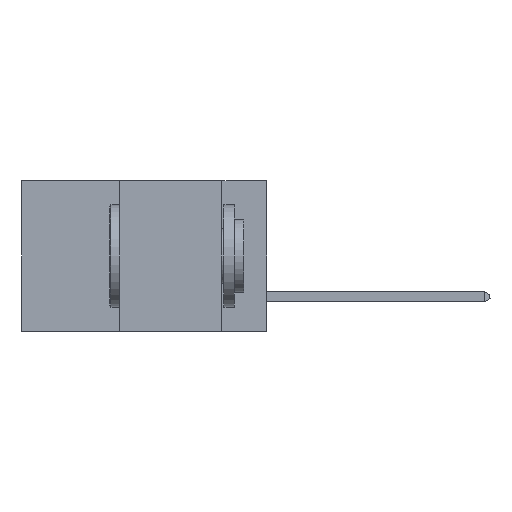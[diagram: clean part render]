
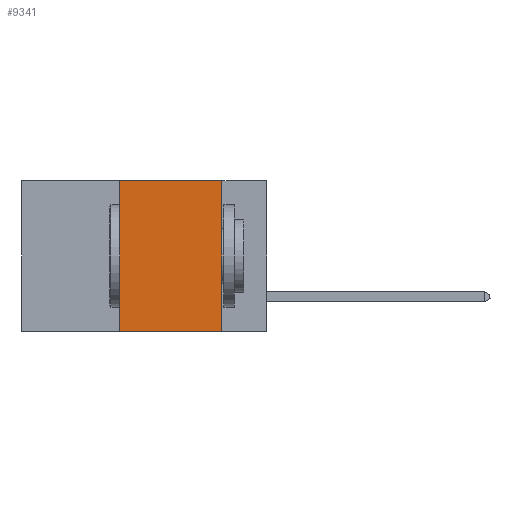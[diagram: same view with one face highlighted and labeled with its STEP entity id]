
A CAD part, left-side view. The second image highlights one B-rep face of the part: STEP entity #9341.
In plain terms, the highlighted planar face has unit normal (-1, 0, 0).
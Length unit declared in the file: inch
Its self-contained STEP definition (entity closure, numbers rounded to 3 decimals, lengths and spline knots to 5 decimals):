
#2614 = FACE_OUTER_BOUND ( 'NONE', #15509, .T. ) ;
#2659 = DIRECTION ( 'NONE',  ( 0., -1., 0. ) ) ;
#3220 = CARTESIAN_POINT ( 'NONE',  ( 0., 0.11, -0.37 ) ) ;
#4090 = DIRECTION ( 'NONE',  ( 0., 0., -1. ) ) ;
#4826 = CARTESIAN_POINT ( 'NONE',  ( 0., 0.36, -0.37 ) ) ;
#5316 = VERTEX_POINT ( 'NONE', #4826 ) ;
#5950 = VECTOR ( 'NONE', #25787, 39.37008 ) ;
#6072 = CARTESIAN_POINT ( 'NONE',  ( 0., 0.6, 0. ) ) ;
#6978 = LINE ( 'NONE', #11052, #22862 ) ;
#7278 = EDGE_CURVE ( 'NONE', #8831, #9367, #6978, .T. ) ;
#8831 = VERTEX_POINT ( 'NONE', #9322 ) ;
#9322 = CARTESIAN_POINT ( 'NONE',  ( 0., 0.36, 0. ) ) ;
#9341 = ADVANCED_FACE ( 'NONE', ( #2614 ), #10230, .F. ) ;
#9367 = VERTEX_POINT ( 'NONE', #18439 ) ;
#10228 = VECTOR ( 'NONE', #10442, 39.37008 ) ;
#10230 = PLANE ( 'NONE',  #13656 ) ;
#10442 = DIRECTION ( 'NONE',  ( 0., 0., 1. ) ) ;
#11052 = CARTESIAN_POINT ( 'NONE',  ( 0., 0.6, 0. ) ) ;
#11776 = EDGE_CURVE ( 'NONE', #5316, #24191, #11885, .T. ) ;
#11885 = LINE ( 'NONE', #15626, #26827 ) ;
#13656 = AXIS2_PLACEMENT_3D ( 'NONE', #6072, #16426, #4090 ) ;
#15509 = EDGE_LOOP ( 'NONE', ( #20911, #16226, #23393, #22900 ) ) ;
#15626 = CARTESIAN_POINT ( 'NONE',  ( 0., 0.6, -0.37 ) ) ;
#15669 = LINE ( 'NONE', #20868, #10228 ) ;
#16226 = ORIENTED_EDGE ( 'NONE', *, *, #7278, .F. ) ;
#16426 = DIRECTION ( 'NONE',  ( 1., 0., 0. ) ) ;
#18439 = CARTESIAN_POINT ( 'NONE',  ( 0., 0.11, 0. ) ) ;
#18896 = LINE ( 'NONE', #25877, #5950 ) ;
#19863 = DIRECTION ( 'NONE',  ( 0., -1., 0. ) ) ;
#20868 = CARTESIAN_POINT ( 'NONE',  ( 0., 0.36, 0. ) ) ;
#20911 = ORIENTED_EDGE ( 'NONE', *, *, #24018, .F. ) ;
#22845 = EDGE_CURVE ( 'NONE', #5316, #8831, #15669, .T. ) ;
#22862 = VECTOR ( 'NONE', #2659, 39.37008 ) ;
#22900 = ORIENTED_EDGE ( 'NONE', *, *, #11776, .T. ) ;
#23393 = ORIENTED_EDGE ( 'NONE', *, *, #22845, .F. ) ;
#24018 = EDGE_CURVE ( 'NONE', #9367, #24191, #18896, .T. ) ;
#24191 = VERTEX_POINT ( 'NONE', #3220 ) ;
#25787 = DIRECTION ( 'NONE',  ( 0., 0., -1. ) ) ;
#25877 = CARTESIAN_POINT ( 'NONE',  ( 0., 0.11, 0. ) ) ;
#26827 = VECTOR ( 'NONE', #19863, 39.37008 ) ;
